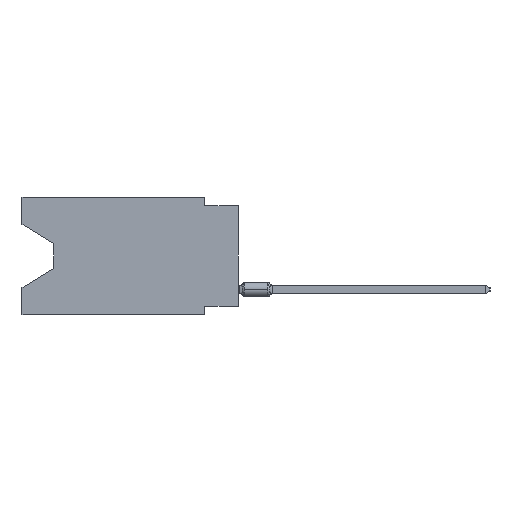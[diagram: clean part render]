
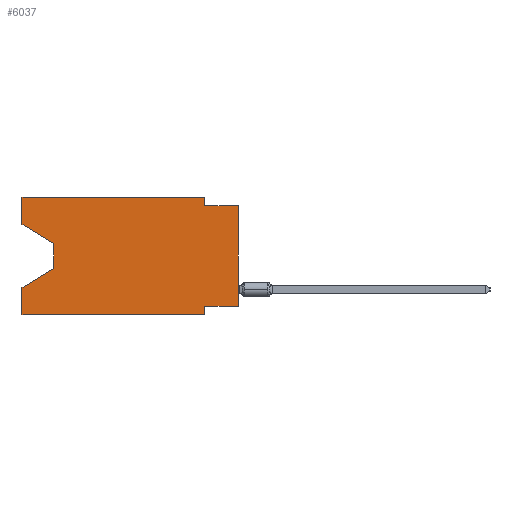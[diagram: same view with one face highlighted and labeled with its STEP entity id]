
A CAD part, left-side view. The second image highlights one B-rep face of the part: STEP entity #6037.
In plain terms, the highlighted planar face has unit normal (-1, 0, 0).
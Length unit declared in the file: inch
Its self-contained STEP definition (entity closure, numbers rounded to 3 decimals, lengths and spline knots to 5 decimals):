
#4498 = EDGE_CURVE ( 'NONE', #22950, #75545, #44280, .T. ) ;
#4796 = CARTESIAN_POINT ( 'NONE',  ( 0., 0.1, -0.025 ) ) ;
#5492 = PLANE ( 'NONE',  #15064 ) ;
#6037 = ADVANCED_FACE ( 'NONE', ( #92736 ), #5492, .F. ) ;
#6141 = CARTESIAN_POINT ( 'NONE',  ( 0., 0., -0.325 ) ) ;
#8260 = ORIENTED_EDGE ( 'NONE', *, *, #58664, .F. ) ;
#8287 = ORIENTED_EDGE ( 'NONE', *, *, #52815, .T. ) ;
#9672 = VECTOR ( 'NONE', #43923, 39.37008 ) ;
#11427 = DIRECTION ( 'NONE',  ( 0., -0.855, -0.519 ) ) ;
#11760 = DIRECTION ( 'NONE',  ( 1., 0., 0. ) ) ;
#14302 = VECTOR ( 'NONE', #15571, 39.37008 ) ;
#14462 = ORIENTED_EDGE ( 'NONE', *, *, #58364, .F. ) ;
#15064 = AXIS2_PLACEMENT_3D ( 'NONE', #37137, #11760, #68320 ) ;
#15336 = VECTOR ( 'NONE', #65627, 39.37008 ) ;
#15571 = DIRECTION ( 'NONE',  ( 0., 0.855, -0.519 ) ) ;
#19222 = LINE ( 'NONE', #19732, #65332 ) ;
#19638 = ORIENTED_EDGE ( 'NONE', *, *, #51036, .F. ) ;
#19732 = CARTESIAN_POINT ( 'NONE',  ( 0., 0.645, -0.08025 ) ) ;
#19862 = VECTOR ( 'NONE', #90717, 39.37008 ) ;
#20976 = CARTESIAN_POINT ( 'NONE',  ( 0., 0.645, -0.35 ) ) ;
#22271 = ORIENTED_EDGE ( 'NONE', *, *, #45086, .F. ) ;
#22809 = CARTESIAN_POINT ( 'NONE',  ( 0., 0.1, -0.35 ) ) ;
#22950 = VERTEX_POINT ( 'NONE', #45619 ) ;
#26179 = CARTESIAN_POINT ( 'NONE',  ( 0., 0.1, 0. ) ) ;
#29244 = ORIENTED_EDGE ( 'NONE', *, *, #53502, .T. ) ;
#29357 = EDGE_CURVE ( 'NONE', #76974, #32045, #19222, .T. ) ;
#32045 = VERTEX_POINT ( 'NONE', #60446 ) ;
#32966 = LINE ( 'NONE', #41249, #35511 ) ;
#33949 = LINE ( 'NONE', #82762, #82277 ) ;
#35511 = VECTOR ( 'NONE', #40223, 39.37008 ) ;
#36660 = LINE ( 'NONE', #82909, #9672 ) ;
#37137 = CARTESIAN_POINT ( 'NONE',  ( 0., 0.645, 0. ) ) ;
#39129 = EDGE_CURVE ( 'NONE', #73896, #87969, #59538, .T. ) ;
#40223 = DIRECTION ( 'NONE',  ( 0., 0., 1. ) ) ;
#41249 = CARTESIAN_POINT ( 'NONE',  ( 0., 0.645, 0. ) ) ;
#41583 = ORIENTED_EDGE ( 'NONE', *, *, #78528, .T. ) ;
#41589 = VERTEX_POINT ( 'NONE', #6141 ) ;
#43276 = DIRECTION ( 'NONE',  ( 0., 0., -1. ) ) ;
#43923 = DIRECTION ( 'NONE',  ( 0., -1., 0. ) ) ;
#44280 = LINE ( 'NONE', #92592, #56267 ) ;
#44811 = DIRECTION ( 'NONE',  ( 0., -1., 0. ) ) ;
#45086 = EDGE_CURVE ( 'NONE', #41589, #46505, #65770, .T. ) ;
#45619 = CARTESIAN_POINT ( 'NONE',  ( 0., 0.645, 0. ) ) ;
#46505 = VERTEX_POINT ( 'NONE', #52901 ) ;
#46708 = CARTESIAN_POINT ( 'NONE',  ( 0., 0.55, -0.212 ) ) ;
#48156 = VERTEX_POINT ( 'NONE', #68588 ) ;
#48429 = ORIENTED_EDGE ( 'NONE', *, *, #39129, .T. ) ;
#49687 = DIRECTION ( 'NONE',  ( 0., 0., 1. ) ) ;
#50343 = CARTESIAN_POINT ( 'NONE',  ( 0., 0., 0. ) ) ;
#51036 = EDGE_CURVE ( 'NONE', #46505, #87969, #62067, .T. ) ;
#52815 = EDGE_CURVE ( 'NONE', #32045, #48156, #33949, .T. ) ;
#52901 = CARTESIAN_POINT ( 'NONE',  ( 0., 0.1, -0.325 ) ) ;
#53502 = EDGE_CURVE ( 'NONE', #48156, #59512, #55529, .T. ) ;
#54000 = EDGE_CURVE ( 'NONE', #75545, #91785, #66159, .T. ) ;
#55529 = LINE ( 'NONE', #46708, #14302 ) ;
#56267 = VECTOR ( 'NONE', #44811, 39.37008 ) ;
#56431 = CARTESIAN_POINT ( 'NONE',  ( 0., 0., -0.025 ) ) ;
#57949 = ORIENTED_EDGE ( 'NONE', *, *, #29357, .T. ) ;
#58364 = EDGE_CURVE ( 'NONE', #76974, #22950, #65258, .T. ) ;
#58664 = EDGE_CURVE ( 'NONE', #73896, #59512, #32966, .T. ) ;
#59512 = VERTEX_POINT ( 'NONE', #63347 ) ;
#59521 = CARTESIAN_POINT ( 'NONE',  ( 0., 0., -0.325 ) ) ;
#59538 = LINE ( 'NONE', #66321, #19862 ) ;
#60446 = CARTESIAN_POINT ( 'NONE',  ( 0., 0.55, -0.138 ) ) ;
#62067 = LINE ( 'NONE', #62571, #95167 ) ;
#62571 = CARTESIAN_POINT ( 'NONE',  ( 0., 0.1, -0.35 ) ) ;
#62853 = ORIENTED_EDGE ( 'NONE', *, *, #54000, .F. ) ;
#63347 = CARTESIAN_POINT ( 'NONE',  ( 0., 0.645, -0.26975 ) ) ;
#65258 = LINE ( 'NONE', #98018, #101878 ) ;
#65332 = VECTOR ( 'NONE', #11427, 39.37008 ) ;
#65529 = VECTOR ( 'NONE', #99693, 39.37008 ) ;
#65627 = DIRECTION ( 'NONE',  ( 0., 0., -1. ) ) ;
#65770 = LINE ( 'NONE', #59521, #102736 ) ;
#66159 = LINE ( 'NONE', #26179, #15336 ) ;
#66321 = CARTESIAN_POINT ( 'NONE',  ( 0., 0.645, -0.35 ) ) ;
#67986 = LINE ( 'NONE', #50343, #65529 ) ;
#68320 = DIRECTION ( 'NONE',  ( 0., 0., -1. ) ) ;
#68588 = CARTESIAN_POINT ( 'NONE',  ( 0., 0.55, -0.212 ) ) ;
#73896 = VERTEX_POINT ( 'NONE', #20976 ) ;
#74882 = ORIENTED_EDGE ( 'NONE', *, *, #95485, .F. ) ;
#75545 = VERTEX_POINT ( 'NONE', #96843 ) ;
#76974 = VERTEX_POINT ( 'NONE', #91482 ) ;
#78528 = EDGE_CURVE ( 'NONE', #41589, #91035, #67986, .T. ) ;
#82277 = VECTOR ( 'NONE', #43276, 39.37008 ) ;
#82762 = CARTESIAN_POINT ( 'NONE',  ( 0., 0.55, -0.138 ) ) ;
#82909 = CARTESIAN_POINT ( 'NONE',  ( 0., 0., -0.025 ) ) ;
#87969 = VERTEX_POINT ( 'NONE', #22809 ) ;
#90690 = EDGE_LOOP ( 'NONE', ( #57949, #8287, #29244, #8260, #48429, #19638, #22271, #41583, #74882, #62853, #96549, #14462 ) ) ;
#90717 = DIRECTION ( 'NONE',  ( 0., -1., 0. ) ) ;
#91035 = VERTEX_POINT ( 'NONE', #56431 ) ;
#91230 = DIRECTION ( 'NONE',  ( 0., 1., 0. ) ) ;
#91482 = CARTESIAN_POINT ( 'NONE',  ( 0., 0.645, -0.08025 ) ) ;
#91785 = VERTEX_POINT ( 'NONE', #4796 ) ;
#92592 = CARTESIAN_POINT ( 'NONE',  ( 0., 0.645, 0. ) ) ;
#92736 = FACE_OUTER_BOUND ( 'NONE', #90690, .T. ) ;
#94801 = DIRECTION ( 'NONE',  ( 0., 0., -1. ) ) ;
#95167 = VECTOR ( 'NONE', #94801, 39.37008 ) ;
#95485 = EDGE_CURVE ( 'NONE', #91785, #91035, #36660, .T. ) ;
#96549 = ORIENTED_EDGE ( 'NONE', *, *, #4498, .F. ) ;
#96843 = CARTESIAN_POINT ( 'NONE',  ( 0., 0.1, 0. ) ) ;
#98018 = CARTESIAN_POINT ( 'NONE',  ( 0., 0.645, 0. ) ) ;
#99693 = DIRECTION ( 'NONE',  ( 0., 0., 1. ) ) ;
#101878 = VECTOR ( 'NONE', #49687, 39.37008 ) ;
#102736 = VECTOR ( 'NONE', #91230, 39.37008 ) ;
